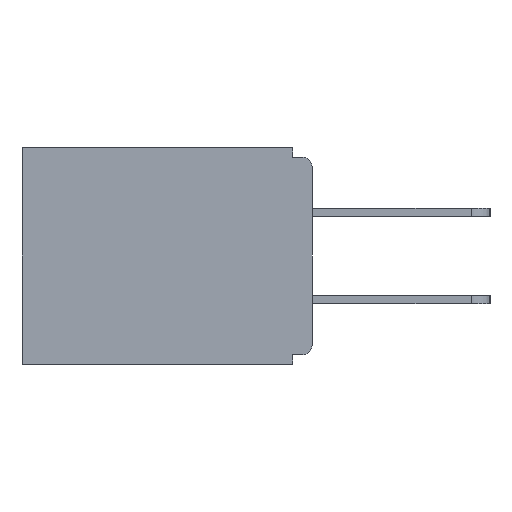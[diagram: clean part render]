
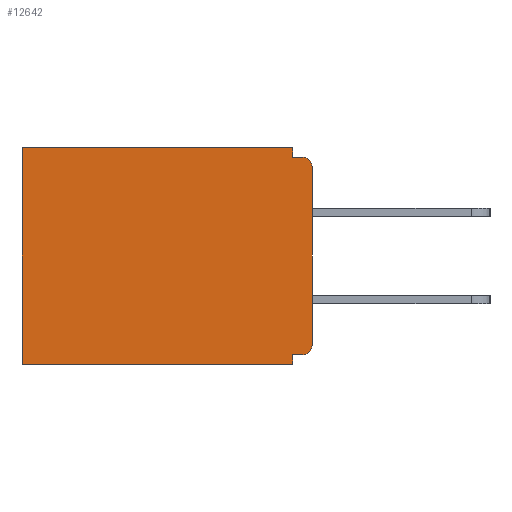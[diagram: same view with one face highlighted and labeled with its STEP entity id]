
A CAD part, left-side view. The second image highlights one B-rep face of the part: STEP entity #12642.
In plain terms, the highlighted planar face has unit normal (-1, 0, 0).
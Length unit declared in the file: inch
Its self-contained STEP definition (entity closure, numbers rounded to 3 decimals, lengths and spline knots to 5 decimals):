
#81 = DIRECTION ( 'NONE',  ( 0., -1., 0. ) ) ;
#414 = ORIENTED_EDGE ( 'NONE', *, *, #3865, .F. ) ;
#559 = VERTEX_POINT ( 'NONE', #14984 ) ;
#604 = CARTESIAN_POINT ( 'NONE',  ( 0.298, 0.031, -0.343 ) ) ;
#1177 = CARTESIAN_POINT ( 'NONE',  ( 0.298, 0.46, 0. ) ) ;
#1340 = CARTESIAN_POINT ( 'NONE',  ( 0.298, 0., -0.03 ) ) ;
#1410 = CARTESIAN_POINT ( 'NONE',  ( 0.298, 0., -0.328 ) ) ;
#1467 = VECTOR ( 'NONE', #4516, 39.37008 ) ;
#1537 = DIRECTION ( 'NONE',  ( 0., 0., -1. ) ) ;
#1609 = VECTOR ( 'NONE', #1537, 39.37008 ) ;
#1766 = DIRECTION ( 'NONE',  ( -1., 0., 0. ) ) ;
#1912 = CARTESIAN_POINT ( 'NONE',  ( 0.298, 0., -0.313 ) ) ;
#2758 = DIRECTION ( 'NONE',  ( -1., 0., 0. ) ) ;
#2886 = VERTEX_POINT ( 'NONE', #9075 ) ;
#3006 = DIRECTION ( 'NONE',  ( 0., 1., 0. ) ) ;
#3229 = VECTOR ( 'NONE', #8415, 39.37008 ) ;
#3474 = CARTESIAN_POINT ( 'NONE',  ( 0.298, 0.46, 0. ) ) ;
#3484 = CARTESIAN_POINT ( 'NONE',  ( 0.298, 0.031, -0.343 ) ) ;
#3541 = EDGE_CURVE ( 'NONE', #4577, #6886, #13985, .T. ) ;
#3662 = PLANE ( 'NONE',  #5267 ) ;
#3827 = VERTEX_POINT ( 'NONE', #11485 ) ;
#3865 = EDGE_CURVE ( 'NONE', #11095, #559, #4305, .T. ) ;
#4305 = LINE ( 'NONE', #3484, #7452 ) ;
#4513 = ORIENTED_EDGE ( 'NONE', *, *, #10529, .T. ) ;
#4516 = DIRECTION ( 'NONE',  ( 0., 0., -1. ) ) ;
#4577 = VERTEX_POINT ( 'NONE', #11116 ) ;
#4644 = ORIENTED_EDGE ( 'NONE', *, *, #3541, .F. ) ;
#4838 = DIRECTION ( 'NONE',  ( 0., 0., -1. ) ) ;
#4928 = CARTESIAN_POINT ( 'NONE',  ( 0.298, 0.031, 0. ) ) ;
#4957 = ORIENTED_EDGE ( 'NONE', *, *, #15161, .T. ) ;
#5267 = AXIS2_PLACEMENT_3D ( 'NONE', #10838, #8793, #4838 ) ;
#5286 = ORIENTED_EDGE ( 'NONE', *, *, #13982, .T. ) ;
#5410 = CARTESIAN_POINT ( 'NONE',  ( 0.298, 0., -0.343 ) ) ;
#5587 = VECTOR ( 'NONE', #12864, 39.37008 ) ;
#5755 = ORIENTED_EDGE ( 'NONE', *, *, #6353, .F. ) ;
#6068 = CARTESIAN_POINT ( 'NONE',  ( 0.298, 0., -0.015 ) ) ;
#6353 = EDGE_CURVE ( 'NONE', #6886, #8055, #12615, .T. ) ;
#6411 = CARTESIAN_POINT ( 'NONE',  ( 0.298, 0., 0. ) ) ;
#6886 = VERTEX_POINT ( 'NONE', #7140 ) ;
#6896 = LINE ( 'NONE', #5410, #14876 ) ;
#7066 = CARTESIAN_POINT ( 'NONE',  ( 0.298, 0.031, -0.343 ) ) ;
#7140 = CARTESIAN_POINT ( 'NONE',  ( 0.298, 0.031, -0.328 ) ) ;
#7452 = VECTOR ( 'NONE', #10466, 39.37008 ) ;
#7698 = VECTOR ( 'NONE', #13063, 39.37008 ) ;
#7874 = DIRECTION ( 'NONE',  ( 0., 0., -1. ) ) ;
#8052 = ORIENTED_EDGE ( 'NONE', *, *, #10698, .F. ) ;
#8055 = VERTEX_POINT ( 'NONE', #604 ) ;
#8118 = EDGE_CURVE ( 'NONE', #13135, #2886, #12739, .T. ) ;
#8240 = CARTESIAN_POINT ( 'NONE',  ( 0.298, 0., 0. ) ) ;
#8314 = FACE_OUTER_BOUND ( 'NONE', #9881, .T. ) ;
#8409 = VERTEX_POINT ( 'NONE', #3474 ) ;
#8415 = DIRECTION ( 'NONE',  ( 0., 1., 0. ) ) ;
#8631 = ORIENTED_EDGE ( 'NONE', *, *, #8118, .T. ) ;
#8793 = DIRECTION ( 'NONE',  ( 1., 0., 0. ) ) ;
#8873 = CARTESIAN_POINT ( 'NONE',  ( 0.298, 0.015, -0.03 ) ) ;
#8973 = LINE ( 'NONE', #6068, #10284 ) ;
#9075 = CARTESIAN_POINT ( 'NONE',  ( 0.298, 0.015, -0.015 ) ) ;
#9304 = AXIS2_PLACEMENT_3D ( 'NONE', #13322, #2758, #11004 ) ;
#9486 = ORIENTED_EDGE ( 'NONE', *, *, #13283, .F. ) ;
#9881 = EDGE_LOOP ( 'NONE', ( #8631, #11811, #414, #4513, #5286, #8052, #5755, #4644, #4957, #9486 ) ) ;
#10027 = EDGE_CURVE ( 'NONE', #559, #2886, #8973, .T. ) ;
#10204 = CIRCLE ( 'NONE', #9304, 0.015 ) ;
#10284 = VECTOR ( 'NONE', #81, 39.37008 ) ;
#10466 = DIRECTION ( 'NONE',  ( 0., 0., -1. ) ) ;
#10529 = EDGE_CURVE ( 'NONE', #11095, #8409, #11737, .T. ) ;
#10698 = EDGE_CURVE ( 'NONE', #8055, #3827, #6896, .T. ) ;
#10735 = LINE ( 'NONE', #6411, #1609 ) ;
#10804 = VERTEX_POINT ( 'NONE', #1912 ) ;
#10838 = CARTESIAN_POINT ( 'NONE',  ( 0.298, 0., 0. ) ) ;
#11004 = DIRECTION ( 'NONE',  ( 0., 0., -1. ) ) ;
#11095 = VERTEX_POINT ( 'NONE', #4928 ) ;
#11116 = CARTESIAN_POINT ( 'NONE',  ( 0.298, 0.015, -0.328 ) ) ;
#11485 = CARTESIAN_POINT ( 'NONE',  ( 0.298, 0.46, -0.343 ) ) ;
#11737 = LINE ( 'NONE', #8240, #5587 ) ;
#11811 = ORIENTED_EDGE ( 'NONE', *, *, #10027, .F. ) ;
#12615 = LINE ( 'NONE', #7066, #1467 ) ;
#12642 = ADVANCED_FACE ( 'NONE', ( #8314 ), #3662, .F. ) ;
#12739 = CIRCLE ( 'NONE', #12992, 0.015 ) ;
#12864 = DIRECTION ( 'NONE',  ( 0., 1., 0. ) ) ;
#12992 = AXIS2_PLACEMENT_3D ( 'NONE', #8873, #1766, #7874 ) ;
#13063 = DIRECTION ( 'NONE',  ( 0., 0., -1. ) ) ;
#13135 = VERTEX_POINT ( 'NONE', #1340 ) ;
#13283 = EDGE_CURVE ( 'NONE', #13135, #10804, #10735, .T. ) ;
#13322 = CARTESIAN_POINT ( 'NONE',  ( 0.298, 0.015, -0.313 ) ) ;
#13674 = LINE ( 'NONE', #1177, #7698 ) ;
#13982 = EDGE_CURVE ( 'NONE', #8409, #3827, #13674, .T. ) ;
#13985 = LINE ( 'NONE', #1410, #3229 ) ;
#14876 = VECTOR ( 'NONE', #3006, 39.37008 ) ;
#14984 = CARTESIAN_POINT ( 'NONE',  ( 0.298, 0.031, -0.015 ) ) ;
#15161 = EDGE_CURVE ( 'NONE', #4577, #10804, #10204, .T. ) ;
